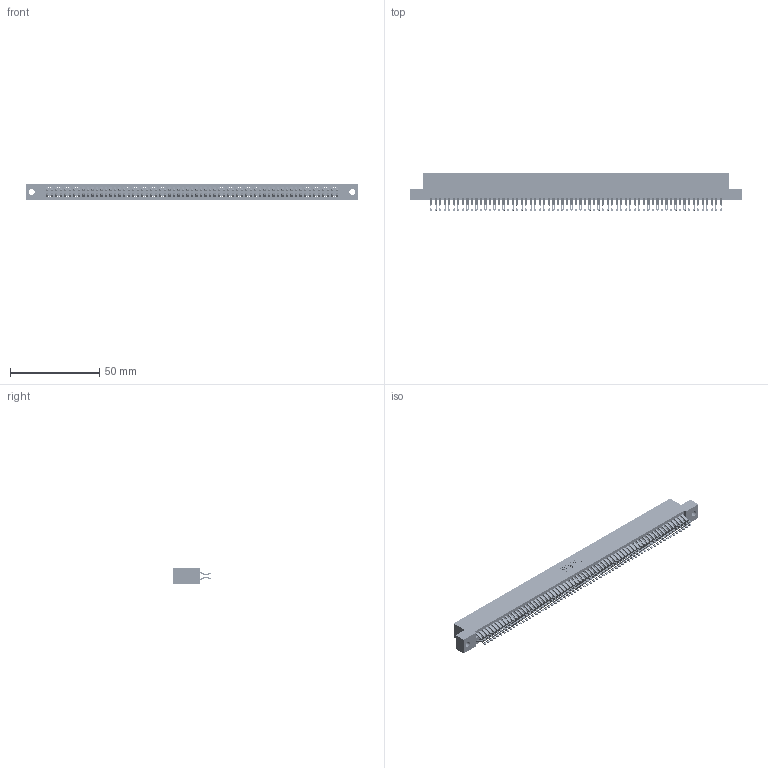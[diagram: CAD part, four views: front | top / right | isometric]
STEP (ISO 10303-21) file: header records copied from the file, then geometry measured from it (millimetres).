
FILE_DESCRIPTION (( 'STEP AP203' ), '1' );
FILE_NAME ('395-130-555-202.STEP', '2019-10-28T23:56:11', ( '' ), ( '' ), 'SwSTEP 2.0', 'SolidWorks 2016', '' );
FILE_SCHEMA (( 'CONFIG_CONTROL_DESIGN' ));
Length unit declared in the file: inch
Products named in the file (3): 345-292-001_555 Tail; 395-130-555-202; 345 Part_Flush Mounting Lugs - 0.128 Dia
Assembly tree (131 placements, depth 2):
  395-130-555-202
    345 Part_Flush Mounting Lugs - 0.128 Dia
    345-292-001_555 Tail  x130
Bounding box: 186.31 x 21.13 x 9.4 mm (x, y, z)
Volume: 18652.1 mm3; surface area: 29055.2 mm2
Topology: 131 solids, 131 shells, 7406 faces, 23351 edges, 15566 vertices
Faces by surface type: plane 4110, cylinder 3296
Entity records: 48233 total; most frequent: CARTESIAN_POINT 8098, ORIENTED_EDGE 8002, DIRECTION 7081, EDGE_CURVE 4001, VECTOR 3589, LINE 3589, VERTEX_POINT 2666, AXIS2_PLACEMENT_3D 1746
